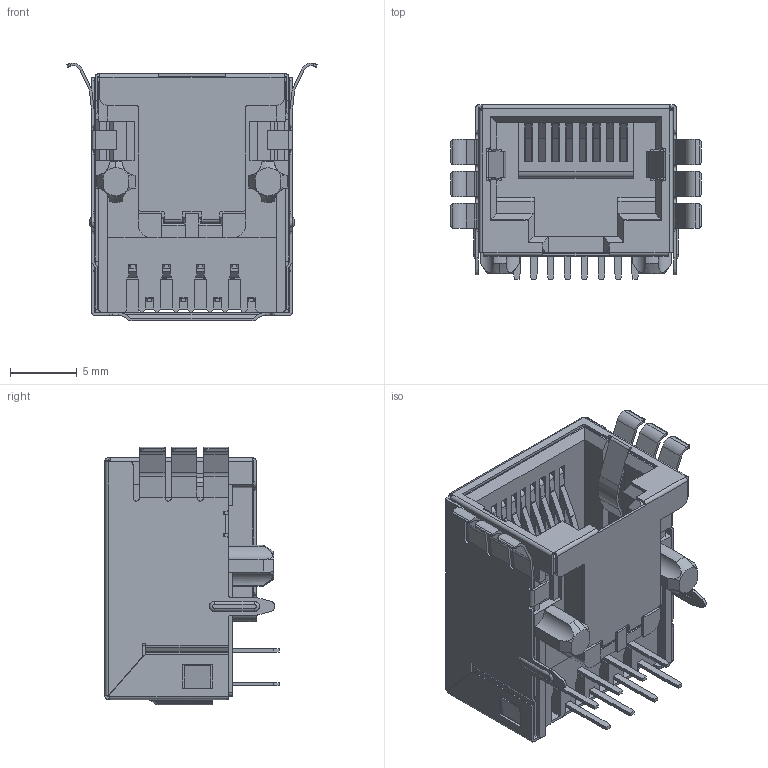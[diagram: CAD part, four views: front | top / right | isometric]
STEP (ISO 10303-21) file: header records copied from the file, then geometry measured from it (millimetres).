
FILE_DESCRIPTION (( 'STEP AP203' ), '1' );
FILE_NAME ('J9Q018862P00202.STEP', '2020-03-17T19:53:21', ( '' ), ( '' ), 'SwSTEP 2.0', 'SolidWorks 2016', '' );
FILE_SCHEMA (( 'CONFIG_CONTROL_DESIGN' ));
Length unit declared in the file: millimetre
Products named in the file (5): 9Q Contacts; J9Q018862P00202; 9Q Shield; 9Q Insulator; 9Q Contact Lock
Assembly tree (4 placements, depth 2):
  J9Q018862P00202
    9Q Insulator
    9Q Contacts
    9Q Contact Lock
    9Q Shield
Bounding box: 18.81 x 13.07 x 19.36 mm (x, y, z)
Volume: 1192.9 mm3; surface area: 4818.3 mm2
Topology: 11 solids, 11 shells, 1339 faces, 3897 edges, 2560 vertices
Faces by surface type: plane 949, cylinder 369, bspline 14, cone 7
Entity records: 44968 total; most frequent: CARTESIAN_POINT 8725, ORIENTED_EDGE 7790, DIRECTION 7135, EDGE_CURVE 3895, VECTOR 3071, LINE 3071, VERTEX_POINT 2560, AXIS2_PLACEMENT_3D 2032
